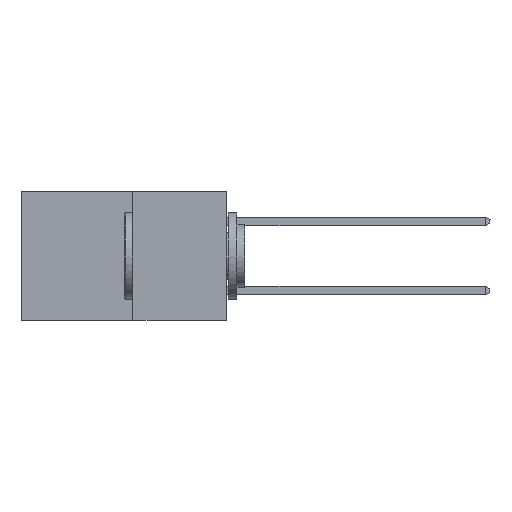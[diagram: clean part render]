
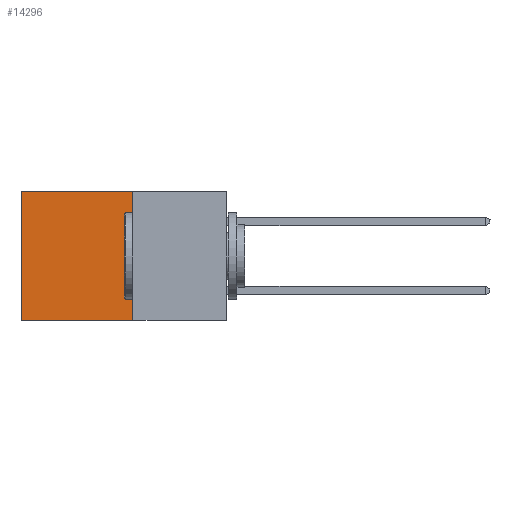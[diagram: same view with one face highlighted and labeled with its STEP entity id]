
A CAD part, left-side view. The second image highlights one B-rep face of the part: STEP entity #14296.
In plain terms, the highlighted planar face has unit normal (-1, 0, 0).
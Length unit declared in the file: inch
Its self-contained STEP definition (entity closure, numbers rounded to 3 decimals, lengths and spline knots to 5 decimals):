
#90 = EDGE_CURVE ( 'NONE', #16080, #15113, #21632, .T. ) ;
#498 = ORIENTED_EDGE ( 'NONE', *, *, #24265, .F. ) ;
#1027 = LINE ( 'NONE', #23710, #15828 ) ;
#1642 = VECTOR ( 'NONE', #2471, 39.37008 ) ;
#2005 = LINE ( 'NONE', #7886, #21839 ) ;
#2471 = DIRECTION ( 'NONE',  ( 0., 0., -1. ) ) ;
#4423 = ORIENTED_EDGE ( 'NONE', *, *, #4641, .F. ) ;
#4552 = DIRECTION ( 'NONE',  ( 1., 0., 0. ) ) ;
#4641 = EDGE_CURVE ( 'NONE', #19404, #5517, #2005, .T. ) ;
#5517 = VERTEX_POINT ( 'NONE', #8867 ) ;
#6444 = CARTESIAN_POINT ( 'NONE',  ( 0.277, 0.27, -0.37 ) ) ;
#6963 = FACE_OUTER_BOUND ( 'NONE', #24620, .T. ) ;
#7886 = CARTESIAN_POINT ( 'NONE',  ( 0.277, 0.27, -0.37 ) ) ;
#8581 = EDGE_CURVE ( 'NONE', #15113, #5517, #11320, .T. ) ;
#8867 = CARTESIAN_POINT ( 'NONE',  ( 0.277, 0.59, -0.37 ) ) ;
#9127 = DIRECTION ( 'NONE',  ( 0., 1., 0. ) ) ;
#10434 = DIRECTION ( 'NONE',  ( 0., 0., -1. ) ) ;
#10636 = CARTESIAN_POINT ( 'NONE',  ( 0.277, 0.59, 0. ) ) ;
#11318 = DIRECTION ( 'NONE',  ( 0., 1., 0. ) ) ;
#11320 = LINE ( 'NONE', #14044, #1642 ) ;
#12100 = AXIS2_PLACEMENT_3D ( 'NONE', #6444, #4552, #18038 ) ;
#12573 = ORIENTED_EDGE ( 'NONE', *, *, #90, .T. ) ;
#13160 = CARTESIAN_POINT ( 'NONE',  ( 0.277, 0.27, 0. ) ) ;
#13186 = CARTESIAN_POINT ( 'NONE',  ( 0.277, 0.27, -0.37 ) ) ;
#14044 = CARTESIAN_POINT ( 'NONE',  ( 0.277, 0.59, -0.37 ) ) ;
#14296 = ADVANCED_FACE ( 'NONE', ( #6963 ), #16118, .F. ) ;
#15113 = VERTEX_POINT ( 'NONE', #10636 ) ;
#15828 = VECTOR ( 'NONE', #10434, 39.37008 ) ;
#16080 = VERTEX_POINT ( 'NONE', #13160 ) ;
#16118 = PLANE ( 'NONE',  #12100 ) ;
#17201 = VECTOR ( 'NONE', #11318, 39.37008 ) ;
#18038 = DIRECTION ( 'NONE',  ( 0., 0., -1. ) ) ;
#18244 = CARTESIAN_POINT ( 'NONE',  ( 0.277, 0.27, 0. ) ) ;
#18591 = ORIENTED_EDGE ( 'NONE', *, *, #8581, .T. ) ;
#19404 = VERTEX_POINT ( 'NONE', #13186 ) ;
#21632 = LINE ( 'NONE', #18244, #17201 ) ;
#21839 = VECTOR ( 'NONE', #9127, 39.37008 ) ;
#23710 = CARTESIAN_POINT ( 'NONE',  ( 0.277, 0.27, -0.37 ) ) ;
#24265 = EDGE_CURVE ( 'NONE', #16080, #19404, #1027, .T. ) ;
#24620 = EDGE_LOOP ( 'NONE', ( #18591, #4423, #498, #12573 ) ) ;
